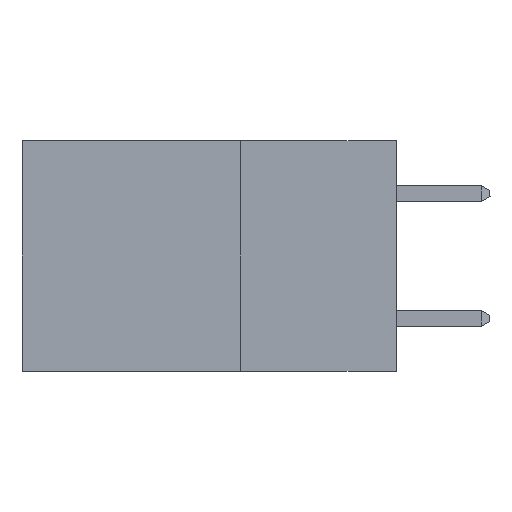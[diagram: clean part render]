
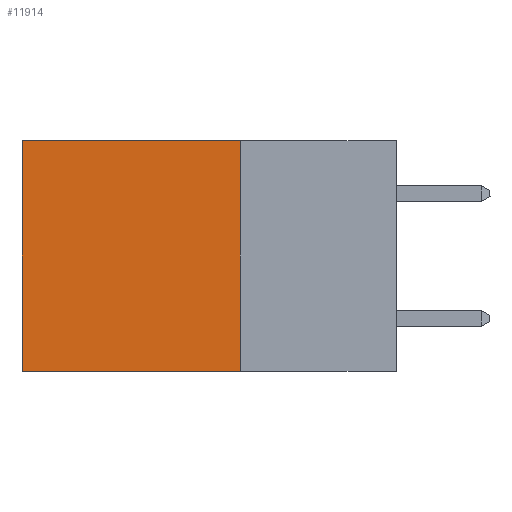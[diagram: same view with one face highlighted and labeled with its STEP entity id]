
A CAD part, left-side view. The second image highlights one B-rep face of the part: STEP entity #11914.
In plain terms, the highlighted planar face has unit normal (-1, 0, 0).
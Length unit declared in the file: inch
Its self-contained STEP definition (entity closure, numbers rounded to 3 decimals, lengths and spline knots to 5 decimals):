
#564 = CARTESIAN_POINT ( 'NONE',  ( 0.298, 0.25, 0. ) ) ;
#731 = LINE ( 'NONE', #760, #2138 ) ;
#760 = CARTESIAN_POINT ( 'NONE',  ( 0.298, 0.25, 0. ) ) ;
#1100 = CARTESIAN_POINT ( 'NONE',  ( 0.298, 0.25, 0. ) ) ;
#1710 = CARTESIAN_POINT ( 'NONE',  ( 0.298, 0.25, 0. ) ) ;
#2138 = VECTOR ( 'NONE', #18123, 39.37008 ) ;
#4158 = LINE ( 'NONE', #7589, #6533 ) ;
#4439 = EDGE_CURVE ( 'NONE', #6136, #23237, #18230, .T. ) ;
#5082 = ORIENTED_EDGE ( 'NONE', *, *, #19995, .T. ) ;
#5997 = VECTOR ( 'NONE', #22334, 39.37008 ) ;
#6136 = VERTEX_POINT ( 'NONE', #24797 ) ;
#6533 = VECTOR ( 'NONE', #16363, 39.37008 ) ;
#7589 = CARTESIAN_POINT ( 'NONE',  ( 0.298, 0.25, -0.37 ) ) ;
#10496 = DIRECTION ( 'NONE',  ( 1., 0., 0. ) ) ;
#10805 = EDGE_CURVE ( 'NONE', #21296, #23237, #4158, .T. ) ;
#10914 = FACE_OUTER_BOUND ( 'NONE', #17612, .T. ) ;
#11468 = EDGE_CURVE ( 'NONE', #22063, #21296, #731, .T. ) ;
#11505 = CARTESIAN_POINT ( 'NONE',  ( 0.298, 0.6, 0. ) ) ;
#11914 = ADVANCED_FACE ( 'NONE', ( #10914 ), #23534, .F. ) ;
#12280 = CARTESIAN_POINT ( 'NONE',  ( 0.298, 0.25, -0.37 ) ) ;
#13817 = AXIS2_PLACEMENT_3D ( 'NONE', #1710, #10496, #25713 ) ;
#15886 = DIRECTION ( 'NONE',  ( 0., 0., -1. ) ) ;
#16363 = DIRECTION ( 'NONE',  ( 0., 1., 0. ) ) ;
#17612 = EDGE_LOOP ( 'NONE', ( #21464, #23370, #19108, #5082 ) ) ;
#18123 = DIRECTION ( 'NONE',  ( 0., 0., -1. ) ) ;
#18230 = LINE ( 'NONE', #11505, #19253 ) ;
#19108 = ORIENTED_EDGE ( 'NONE', *, *, #11468, .F. ) ;
#19253 = VECTOR ( 'NONE', #15886, 39.37008 ) ;
#19995 = EDGE_CURVE ( 'NONE', #22063, #6136, #24012, .T. ) ;
#21296 = VERTEX_POINT ( 'NONE', #12280 ) ;
#21464 = ORIENTED_EDGE ( 'NONE', *, *, #4439, .T. ) ;
#22063 = VERTEX_POINT ( 'NONE', #1100 ) ;
#22334 = DIRECTION ( 'NONE',  ( 0., 1., 0. ) ) ;
#23237 = VERTEX_POINT ( 'NONE', #24207 ) ;
#23370 = ORIENTED_EDGE ( 'NONE', *, *, #10805, .F. ) ;
#23534 = PLANE ( 'NONE',  #13817 ) ;
#24012 = LINE ( 'NONE', #564, #5997 ) ;
#24207 = CARTESIAN_POINT ( 'NONE',  ( 0.298, 0.6, -0.37 ) ) ;
#24797 = CARTESIAN_POINT ( 'NONE',  ( 0.298, 0.6, 0. ) ) ;
#25713 = DIRECTION ( 'NONE',  ( 0., 0., -1. ) ) ;
